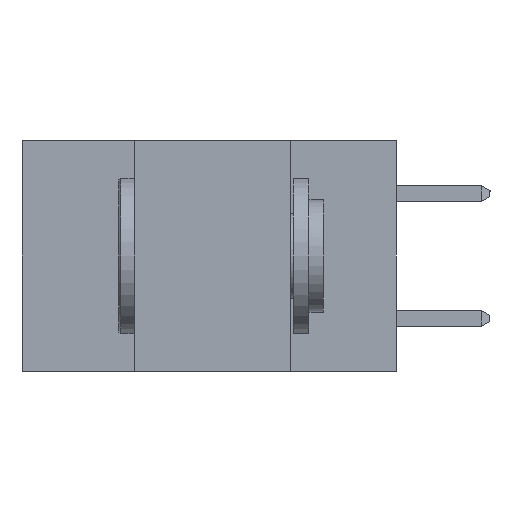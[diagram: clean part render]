
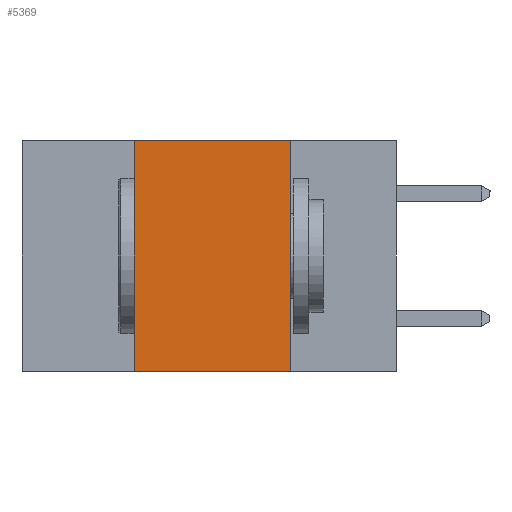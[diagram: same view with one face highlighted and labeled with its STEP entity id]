
A CAD part, left-side view. The second image highlights one B-rep face of the part: STEP entity #5369.
In plain terms, the highlighted planar face has unit normal (-1, 0, 0).
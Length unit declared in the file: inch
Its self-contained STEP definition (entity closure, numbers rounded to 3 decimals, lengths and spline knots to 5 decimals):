
#2092 = CARTESIAN_POINT ( 'NONE',  ( 0., 0.17, -0.37 ) ) ;
#2236 = DIRECTION ( 'NONE',  ( 0., -1., 0. ) ) ;
#2359 = VECTOR ( 'NONE', #6235, 39.37008 ) ;
#2457 = FACE_OUTER_BOUND ( 'NONE', #9128, .T. ) ;
#2889 = LINE ( 'NONE', #7037, #12473 ) ;
#3159 = ORIENTED_EDGE ( 'NONE', *, *, #3363, .T. ) ;
#3230 = VERTEX_POINT ( 'NONE', #6172 ) ;
#3345 = ORIENTED_EDGE ( 'NONE', *, *, #9446, .F. ) ;
#3363 = EDGE_CURVE ( 'NONE', #3230, #9742, #4404, .T. ) ;
#4404 = LINE ( 'NONE', #6238, #4717 ) ;
#4507 = VERTEX_POINT ( 'NONE', #5872 ) ;
#4717 = VECTOR ( 'NONE', #2236, 39.37008 ) ;
#5151 = DIRECTION ( 'NONE',  ( 0., -1., 0. ) ) ;
#5184 = VECTOR ( 'NONE', #5151, 39.37008 ) ;
#5369 = ADVANCED_FACE ( 'NONE', ( #2457 ), #7636, .F. ) ;
#5872 = CARTESIAN_POINT ( 'NONE',  ( 0., 0.17, 0. ) ) ;
#6172 = CARTESIAN_POINT ( 'NONE',  ( 0., 0.42, -0.37 ) ) ;
#6235 = DIRECTION ( 'NONE',  ( 0., 0., -1. ) ) ;
#6238 = CARTESIAN_POINT ( 'NONE',  ( 0., 0.6, -0.37 ) ) ;
#6606 = DIRECTION ( 'NONE',  ( 0., 0., -1. ) ) ;
#7037 = CARTESIAN_POINT ( 'NONE',  ( 0., 0.42, -0.37 ) ) ;
#7636 = PLANE ( 'NONE',  #8283 ) ;
#7639 = ORIENTED_EDGE ( 'NONE', *, *, #13303, .F. ) ;
#8283 = AXIS2_PLACEMENT_3D ( 'NONE', #12747, #10505, #6606 ) ;
#8635 = VERTEX_POINT ( 'NONE', #9406 ) ;
#9128 = EDGE_LOOP ( 'NONE', ( #11876, #7639, #3345, #3159 ) ) ;
#9210 = CARTESIAN_POINT ( 'NONE',  ( 0., 0.6, 0. ) ) ;
#9406 = CARTESIAN_POINT ( 'NONE',  ( 0., 0.42, 0. ) ) ;
#9446 = EDGE_CURVE ( 'NONE', #3230, #8635, #2889, .T. ) ;
#9742 = VERTEX_POINT ( 'NONE', #9906 ) ;
#9906 = CARTESIAN_POINT ( 'NONE',  ( 0., 0.17, -0.37 ) ) ;
#10456 = EDGE_CURVE ( 'NONE', #4507, #9742, #13276, .T. ) ;
#10505 = DIRECTION ( 'NONE',  ( 1., 0., 0. ) ) ;
#11213 = DIRECTION ( 'NONE',  ( 0., 0., 1. ) ) ;
#11317 = LINE ( 'NONE', #9210, #5184 ) ;
#11876 = ORIENTED_EDGE ( 'NONE', *, *, #10456, .F. ) ;
#12473 = VECTOR ( 'NONE', #11213, 39.37008 ) ;
#12747 = CARTESIAN_POINT ( 'NONE',  ( 0., 0.6, 0. ) ) ;
#13276 = LINE ( 'NONE', #2092, #2359 ) ;
#13303 = EDGE_CURVE ( 'NONE', #8635, #4507, #11317, .T. ) ;
